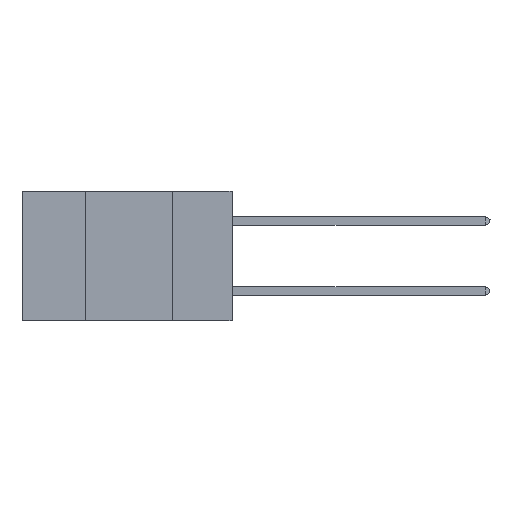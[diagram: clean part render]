
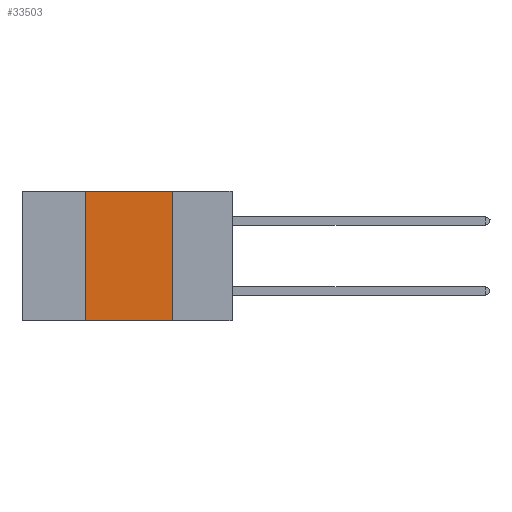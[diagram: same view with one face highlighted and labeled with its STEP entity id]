
A CAD part, left-side view. The second image highlights one B-rep face of the part: STEP entity #33503.
In plain terms, the highlighted planar face has unit normal (-1, 0, 0).
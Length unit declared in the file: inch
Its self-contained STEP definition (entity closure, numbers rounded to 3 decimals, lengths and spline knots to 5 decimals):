
#618 = VERTEX_POINT ( 'NONE', #13541 ) ;
#715 = VERTEX_POINT ( 'NONE', #14128 ) ;
#1661 = FACE_OUTER_BOUND ( 'NONE', #25116, .T. ) ;
#2355 = DIRECTION ( 'NONE',  ( 0., 0., 1. ) ) ;
#3907 = ORIENTED_EDGE ( 'NONE', *, *, #27920, .F. ) ;
#4598 = LINE ( 'NONE', #38483, #30952 ) ;
#6357 = CARTESIAN_POINT ( 'NONE',  ( 0., 0.42, -0.37 ) ) ;
#6906 = LINE ( 'NONE', #10121, #9391 ) ;
#9391 = VECTOR ( 'NONE', #16172, 39.37008 ) ;
#10121 = CARTESIAN_POINT ( 'NONE',  ( 0., 0.6, 0. ) ) ;
#10938 = CARTESIAN_POINT ( 'NONE',  ( 0., 0.6, 0. ) ) ;
#13541 = CARTESIAN_POINT ( 'NONE',  ( 0., 0.17, 0. ) ) ;
#13553 = ORIENTED_EDGE ( 'NONE', *, *, #38876, .F. ) ;
#14128 = CARTESIAN_POINT ( 'NONE',  ( 0., 0.17, -0.37 ) ) ;
#14677 = EDGE_CURVE ( 'NONE', #16853, #715, #4598, .T. ) ;
#15994 = DIRECTION ( 'NONE',  ( 0., 0., -1. ) ) ;
#16172 = DIRECTION ( 'NONE',  ( 0., -1., 0. ) ) ;
#16853 = VERTEX_POINT ( 'NONE', #6357 ) ;
#16973 = DIRECTION ( 'NONE',  ( 0., 0., -1. ) ) ;
#18421 = CARTESIAN_POINT ( 'NONE',  ( 0., 0.17, 0. ) ) ;
#20700 = LINE ( 'NONE', #33016, #27256 ) ;
#25116 = EDGE_LOOP ( 'NONE', ( #38847, #3907, #13553, #32357 ) ) ;
#25874 = DIRECTION ( 'NONE',  ( 1., 0., 0. ) ) ;
#26443 = VECTOR ( 'NONE', #15994, 39.37008 ) ;
#27191 = VERTEX_POINT ( 'NONE', #39273 ) ;
#27256 = VECTOR ( 'NONE', #2355, 39.37008 ) ;
#27741 = AXIS2_PLACEMENT_3D ( 'NONE', #10938, #25874, #16973 ) ;
#27920 = EDGE_CURVE ( 'NONE', #27191, #618, #6906, .T. ) ;
#30952 = VECTOR ( 'NONE', #31833, 39.37008 ) ;
#31833 = DIRECTION ( 'NONE',  ( 0., -1., 0. ) ) ;
#32357 = ORIENTED_EDGE ( 'NONE', *, *, #14677, .T. ) ;
#33016 = CARTESIAN_POINT ( 'NONE',  ( 0., 0.42, 0. ) ) ;
#33445 = EDGE_CURVE ( 'NONE', #618, #715, #34371, .T. ) ;
#33503 = ADVANCED_FACE ( 'NONE', ( #1661 ), #35575, .F. ) ;
#34371 = LINE ( 'NONE', #18421, #26443 ) ;
#35575 = PLANE ( 'NONE',  #27741 ) ;
#38483 = CARTESIAN_POINT ( 'NONE',  ( 0., 0.6, -0.37 ) ) ;
#38847 = ORIENTED_EDGE ( 'NONE', *, *, #33445, .F. ) ;
#38876 = EDGE_CURVE ( 'NONE', #16853, #27191, #20700, .T. ) ;
#39273 = CARTESIAN_POINT ( 'NONE',  ( 0., 0.42, 0. ) ) ;
